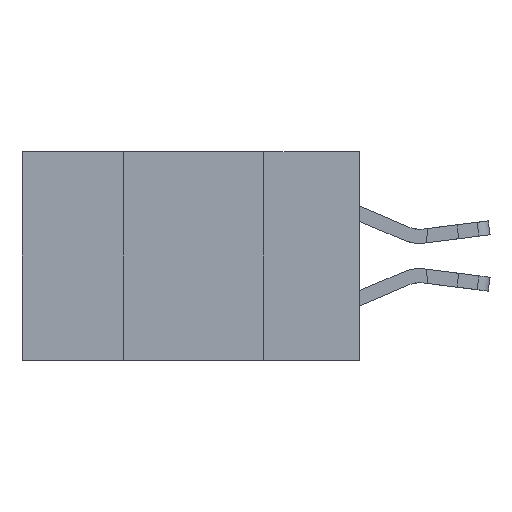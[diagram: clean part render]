
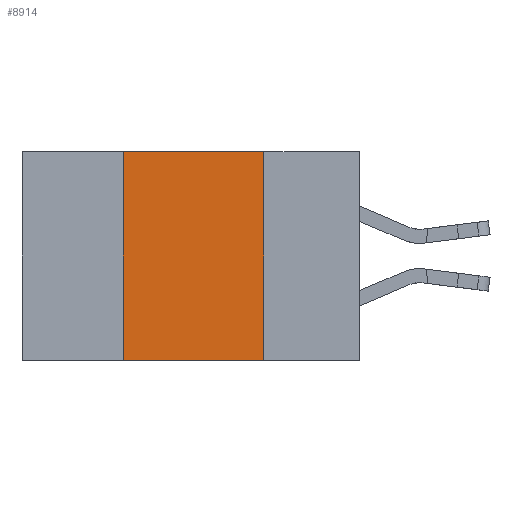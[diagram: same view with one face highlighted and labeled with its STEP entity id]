
A CAD part, left-side view. The second image highlights one B-rep face of the part: STEP entity #8914.
In plain terms, the highlighted planar face has unit normal (-1, 0, 0).
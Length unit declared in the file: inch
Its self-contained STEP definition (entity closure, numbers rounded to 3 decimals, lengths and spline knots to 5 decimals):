
#48 = AXIS2_PLACEMENT_3D ( 'NONE', #26788, #1736, #20582 ) ;
#1103 = EDGE_LOOP ( 'NONE', ( #25471, #18753, #5244, #11389 ) ) ;
#1472 = DIRECTION ( 'NONE',  ( 0., 0., 1. ) ) ;
#1736 = DIRECTION ( 'NONE',  ( 1., 0., 0. ) ) ;
#2049 = CARTESIAN_POINT ( 'NONE',  ( 0., 0.6, 0. ) ) ;
#2776 = VECTOR ( 'NONE', #8373, 39.37008 ) ;
#2792 = LINE ( 'NONE', #6856, #9734 ) ;
#3609 = EDGE_CURVE ( 'NONE', #5031, #14674, #20413, .T. ) ;
#4181 = EDGE_CURVE ( 'NONE', #10486, #6233, #2792, .T. ) ;
#5031 = VERTEX_POINT ( 'NONE', #6408 ) ;
#5244 = ORIENTED_EDGE ( 'NONE', *, *, #3609, .F. ) ;
#6233 = VERTEX_POINT ( 'NONE', #17893 ) ;
#6408 = CARTESIAN_POINT ( 'NONE',  ( 0., 0.42, -0.37 ) ) ;
#6856 = CARTESIAN_POINT ( 'NONE',  ( 0., 0.17, 0. ) ) ;
#7401 = LINE ( 'NONE', #10216, #2776 ) ;
#7937 = PLANE ( 'NONE',  #48 ) ;
#8373 = DIRECTION ( 'NONE',  ( 0., -1., 0. ) ) ;
#8914 = ADVANCED_FACE ( 'NONE', ( #11781 ), #7937, .F. ) ;
#9682 = EDGE_CURVE ( 'NONE', #14674, #10486, #13412, .T. ) ;
#9734 = VECTOR ( 'NONE', #15137, 39.37008 ) ;
#9764 = VECTOR ( 'NONE', #1472, 39.37008 ) ;
#10216 = CARTESIAN_POINT ( 'NONE',  ( 0., 0.6, -0.37 ) ) ;
#10486 = VERTEX_POINT ( 'NONE', #25729 ) ;
#11389 = ORIENTED_EDGE ( 'NONE', *, *, #18087, .T. ) ;
#11781 = FACE_OUTER_BOUND ( 'NONE', #1103, .T. ) ;
#13412 = LINE ( 'NONE', #2049, #16420 ) ;
#14643 = DIRECTION ( 'NONE',  ( 0., -1., 0. ) ) ;
#14674 = VERTEX_POINT ( 'NONE', #20665 ) ;
#15137 = DIRECTION ( 'NONE',  ( 0., 0., -1. ) ) ;
#16420 = VECTOR ( 'NONE', #14643, 39.37008 ) ;
#17893 = CARTESIAN_POINT ( 'NONE',  ( 0., 0.17, -0.37 ) ) ;
#18087 = EDGE_CURVE ( 'NONE', #5031, #6233, #7401, .T. ) ;
#18753 = ORIENTED_EDGE ( 'NONE', *, *, #9682, .F. ) ;
#20413 = LINE ( 'NONE', #26716, #9764 ) ;
#20582 = DIRECTION ( 'NONE',  ( 0., 0., -1. ) ) ;
#20665 = CARTESIAN_POINT ( 'NONE',  ( 0., 0.42, 0. ) ) ;
#25471 = ORIENTED_EDGE ( 'NONE', *, *, #4181, .F. ) ;
#25729 = CARTESIAN_POINT ( 'NONE',  ( 0., 0.17, 0. ) ) ;
#26716 = CARTESIAN_POINT ( 'NONE',  ( 0., 0.42, 0. ) ) ;
#26788 = CARTESIAN_POINT ( 'NONE',  ( 0., 0.6, 0. ) ) ;
